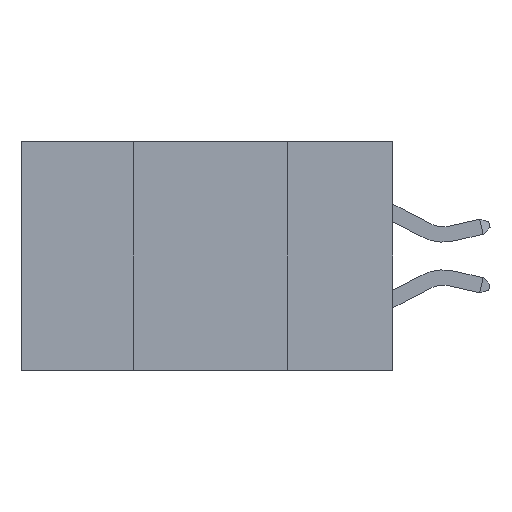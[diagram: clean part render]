
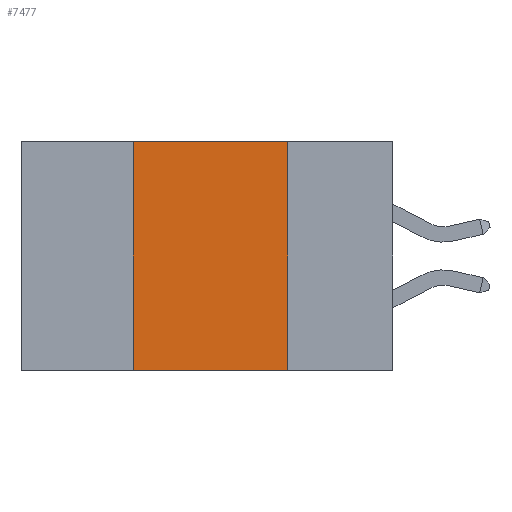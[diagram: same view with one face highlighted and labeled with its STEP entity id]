
A CAD part, left-side view. The second image highlights one B-rep face of the part: STEP entity #7477.
In plain terms, the highlighted planar face has unit normal (-1, 0, 0).
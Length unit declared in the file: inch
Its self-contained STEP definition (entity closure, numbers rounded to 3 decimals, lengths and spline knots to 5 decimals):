
#1659 = VERTEX_POINT ( 'NONE', #12980 ) ;
#1831 = VECTOR ( 'NONE', #14204, 39.37008 ) ;
#2822 = CARTESIAN_POINT ( 'NONE',  ( 0., 0.6, 0. ) ) ;
#2921 = CARTESIAN_POINT ( 'NONE',  ( 0., 0.6, -0.37 ) ) ;
#3168 = ORIENTED_EDGE ( 'NONE', *, *, #3269, .F. ) ;
#3269 = EDGE_CURVE ( 'NONE', #1659, #13934, #11805, .T. ) ;
#3927 = FACE_OUTER_BOUND ( 'NONE', #8185, .T. ) ;
#4638 = CARTESIAN_POINT ( 'NONE',  ( 0., 0.42, -0.37 ) ) ;
#4983 = DIRECTION ( 'NONE',  ( 1., 0., 0. ) ) ;
#5182 = DIRECTION ( 'NONE',  ( 0., -1., 0. ) ) ;
#5758 = CARTESIAN_POINT ( 'NONE',  ( 0., 0.17, 0. ) ) ;
#5924 = EDGE_CURVE ( 'NONE', #14770, #9630, #10906, .T. ) ;
#5965 = LINE ( 'NONE', #7243, #7807 ) ;
#6936 = EDGE_CURVE ( 'NONE', #13934, #9630, #9223, .T. ) ;
#7243 = CARTESIAN_POINT ( 'NONE',  ( 0., 0.42, 0. ) ) ;
#7477 = ADVANCED_FACE ( 'NONE', ( #3927 ), #14020, .F. ) ;
#7519 = VECTOR ( 'NONE', #9290, 39.37008 ) ;
#7807 = VECTOR ( 'NONE', #8382, 39.37008 ) ;
#8013 = AXIS2_PLACEMENT_3D ( 'NONE', #8527, #4983, #8378 ) ;
#8185 = EDGE_LOOP ( 'NONE', ( #8254, #3168, #10380, #11940 ) ) ;
#8254 = ORIENTED_EDGE ( 'NONE', *, *, #6936, .F. ) ;
#8378 = DIRECTION ( 'NONE',  ( 0., 0., -1. ) ) ;
#8382 = DIRECTION ( 'NONE',  ( 0., 0., 1. ) ) ;
#8527 = CARTESIAN_POINT ( 'NONE',  ( 0., 0.6, 0. ) ) ;
#8680 = EDGE_CURVE ( 'NONE', #14770, #1659, #5965, .T. ) ;
#9223 = LINE ( 'NONE', #5758, #7519 ) ;
#9290 = DIRECTION ( 'NONE',  ( 0., 0., -1. ) ) ;
#9630 = VERTEX_POINT ( 'NONE', #13916 ) ;
#10143 = VECTOR ( 'NONE', #5182, 39.37008 ) ;
#10380 = ORIENTED_EDGE ( 'NONE', *, *, #8680, .F. ) ;
#10856 = CARTESIAN_POINT ( 'NONE',  ( 0., 0.17, 0. ) ) ;
#10906 = LINE ( 'NONE', #2921, #10143 ) ;
#11805 = LINE ( 'NONE', #2822, #1831 ) ;
#11940 = ORIENTED_EDGE ( 'NONE', *, *, #5924, .T. ) ;
#12980 = CARTESIAN_POINT ( 'NONE',  ( 0., 0.42, 0. ) ) ;
#13916 = CARTESIAN_POINT ( 'NONE',  ( 0., 0.17, -0.37 ) ) ;
#13934 = VERTEX_POINT ( 'NONE', #10856 ) ;
#14020 = PLANE ( 'NONE',  #8013 ) ;
#14204 = DIRECTION ( 'NONE',  ( 0., -1., 0. ) ) ;
#14770 = VERTEX_POINT ( 'NONE', #4638 ) ;
